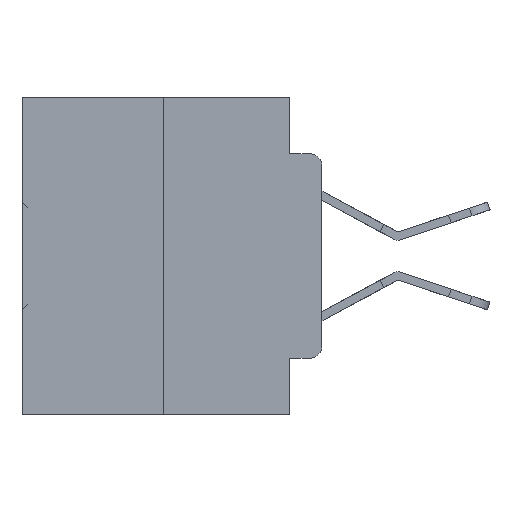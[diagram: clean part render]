
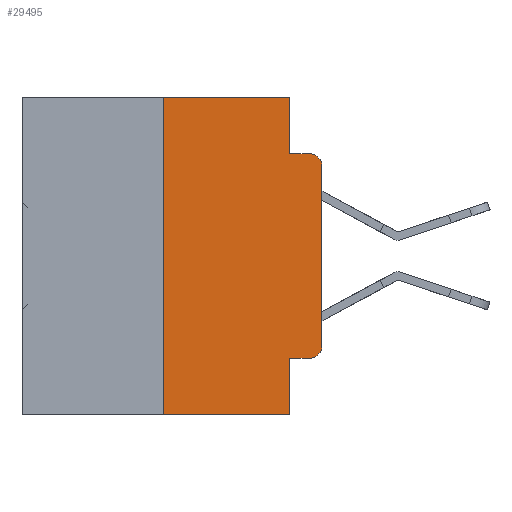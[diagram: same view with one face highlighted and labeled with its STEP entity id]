
A CAD part, left-side view. The second image highlights one B-rep face of the part: STEP entity #29495.
In plain terms, the highlighted planar face has unit normal (-1, 0, 0).
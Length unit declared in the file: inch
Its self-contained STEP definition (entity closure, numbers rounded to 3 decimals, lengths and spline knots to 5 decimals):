
#319 = CARTESIAN_POINT ( 'NONE',  ( 0., 0.051, -0.5 ) ) ;
#462 = VERTEX_POINT ( 'NONE', #13307 ) ;
#950 = VERTEX_POINT ( 'NONE', #319 ) ;
#994 = DIRECTION ( 'NONE',  ( -1., 0., 0. ) ) ;
#1073 = EDGE_CURVE ( 'NONE', #1908, #5815, #4801, .T. ) ;
#1793 = EDGE_CURVE ( 'NONE', #462, #9292, #20117, .T. ) ;
#1815 = LINE ( 'NONE', #3120, #23038 ) ;
#1858 = VERTEX_POINT ( 'NONE', #3463 ) ;
#1908 = VERTEX_POINT ( 'NONE', #36697 ) ;
#2003 = CARTESIAN_POINT ( 'NONE',  ( 0., 0.02, -0.4115 ) ) ;
#2181 = EDGE_CURVE ( 'NONE', #5815, #10513, #35860, .T. ) ;
#3120 = CARTESIAN_POINT ( 'NONE',  ( 0., 0.473, -0.5 ) ) ;
#3243 = CARTESIAN_POINT ( 'NONE',  ( 0., 0.02, -0.3915 ) ) ;
#3463 = CARTESIAN_POINT ( 'NONE',  ( 0., 0., -0.1085 ) ) ;
#3665 = CARTESIAN_POINT ( 'NONE',  ( 0., 0.051, -0.4115 ) ) ;
#3988 = DIRECTION ( 'NONE',  ( 0., 0., 1. ) ) ;
#4154 = LINE ( 'NONE', #35798, #26167 ) ;
#4536 = VECTOR ( 'NONE', #30514, 39.37008 ) ;
#4801 = LINE ( 'NONE', #12631, #35248 ) ;
#5329 = LINE ( 'NONE', #26248, #19744 ) ;
#5815 = VERTEX_POINT ( 'NONE', #7677 ) ;
#6037 = DIRECTION ( 'NONE',  ( 0., -1., 0. ) ) ;
#6159 = DIRECTION ( 'NONE',  ( 0., 0., -1. ) ) ;
#7382 = CARTESIAN_POINT ( 'NONE',  ( 0., 0., -0.3915 ) ) ;
#7677 = CARTESIAN_POINT ( 'NONE',  ( 0., 0.25, 0. ) ) ;
#7715 = CIRCLE ( 'NONE', #22356, 0.02 ) ;
#7912 = EDGE_CURVE ( 'NONE', #10513, #11655, #4154, .T. ) ;
#8356 = CARTESIAN_POINT ( 'NONE',  ( 0., 0.051, 0. ) ) ;
#9292 = VERTEX_POINT ( 'NONE', #2003 ) ;
#10027 = LINE ( 'NONE', #8356, #32860 ) ;
#10513 = VERTEX_POINT ( 'NONE', #33299 ) ;
#10878 = ORIENTED_EDGE ( 'NONE', *, *, #2181, .F. ) ;
#11516 = CARTESIAN_POINT ( 'NONE',  ( 0., 0.051, -0.0885 ) ) ;
#11655 = VERTEX_POINT ( 'NONE', #11516 ) ;
#11855 = ORIENTED_EDGE ( 'NONE', *, *, #34479, .T. ) ;
#11973 = DIRECTION ( 'NONE',  ( 0., 0., 1. ) ) ;
#12333 = ORIENTED_EDGE ( 'NONE', *, *, #1073, .F. ) ;
#12481 = VECTOR ( 'NONE', #24177, 39.37008 ) ;
#12631 = CARTESIAN_POINT ( 'NONE',  ( 0., 0.25, 0. ) ) ;
#13307 = CARTESIAN_POINT ( 'NONE',  ( 0., 0.051, -0.4115 ) ) ;
#13730 = CARTESIAN_POINT ( 'NONE',  ( 0., 0.051, -0.0885 ) ) ;
#14408 = EDGE_LOOP ( 'NONE', ( #31384, #11855, #27970, #23119, #10878, #12333, #22554, #16230, #30542, #15329 ) ) ;
#14472 = FACE_OUTER_BOUND ( 'NONE', #14408, .T. ) ;
#14640 = EDGE_CURVE ( 'NONE', #11655, #15395, #29406, .T. ) ;
#14835 = DIRECTION ( 'NONE',  ( 1., 0., 0. ) ) ;
#15329 = ORIENTED_EDGE ( 'NONE', *, *, #29477, .T. ) ;
#15395 = VERTEX_POINT ( 'NONE', #28304 ) ;
#16230 = ORIENTED_EDGE ( 'NONE', *, *, #28770, .F. ) ;
#16600 = DIRECTION ( 'NONE',  ( 0., -1., 0. ) ) ;
#17180 = AXIS2_PLACEMENT_3D ( 'NONE', #18280, #994, #21189 ) ;
#18153 = VERTEX_POINT ( 'NONE', #7382 ) ;
#18280 = CARTESIAN_POINT ( 'NONE',  ( 0., 0.02, -0.1085 ) ) ;
#18786 = DIRECTION ( 'NONE',  ( 0., 0., -1. ) ) ;
#19744 = VECTOR ( 'NONE', #11973, 39.37008 ) ;
#20117 = LINE ( 'NONE', #3665, #12481 ) ;
#21189 = DIRECTION ( 'NONE',  ( 0., 0., -1. ) ) ;
#22340 = EDGE_CURVE ( 'NONE', #18153, #1858, #5329, .T. ) ;
#22356 = AXIS2_PLACEMENT_3D ( 'NONE', #3243, #23403, #6159 ) ;
#22554 = ORIENTED_EDGE ( 'NONE', *, *, #29467, .T. ) ;
#22942 = CIRCLE ( 'NONE', #17180, 0.02 ) ;
#23038 = VECTOR ( 'NONE', #6037, 39.37008 ) ;
#23119 = ORIENTED_EDGE ( 'NONE', *, *, #7912, .F. ) ;
#23403 = DIRECTION ( 'NONE',  ( -1., 0., 0. ) ) ;
#24177 = DIRECTION ( 'NONE',  ( 0., -1., 0. ) ) ;
#25536 = DIRECTION ( 'NONE',  ( 0., 0., -1. ) ) ;
#26167 = VECTOR ( 'NONE', #18786, 39.37008 ) ;
#26241 = CARTESIAN_POINT ( 'NONE',  ( 0., 0.473, 0. ) ) ;
#26248 = CARTESIAN_POINT ( 'NONE',  ( 0., 0., 0. ) ) ;
#27970 = ORIENTED_EDGE ( 'NONE', *, *, #14640, .F. ) ;
#28304 = CARTESIAN_POINT ( 'NONE',  ( 0., 0.02, -0.0885 ) ) ;
#28770 = EDGE_CURVE ( 'NONE', #462, #950, #10027, .T. ) ;
#29406 = LINE ( 'NONE', #13730, #36908 ) ;
#29467 = EDGE_CURVE ( 'NONE', #1908, #950, #1815, .T. ) ;
#29477 = EDGE_CURVE ( 'NONE', #9292, #18153, #7715, .T. ) ;
#29495 = ADVANCED_FACE ( 'NONE', ( #14472 ), #31972, .F. ) ;
#30514 = DIRECTION ( 'NONE',  ( 0., -1., 0. ) ) ;
#30542 = ORIENTED_EDGE ( 'NONE', *, *, #1793, .T. ) ;
#31384 = ORIENTED_EDGE ( 'NONE', *, *, #22340, .T. ) ;
#31972 = PLANE ( 'NONE',  #33787 ) ;
#32860 = VECTOR ( 'NONE', #25536, 39.37008 ) ;
#33299 = CARTESIAN_POINT ( 'NONE',  ( 0., 0.051, 0. ) ) ;
#33787 = AXIS2_PLACEMENT_3D ( 'NONE', #26241, #14835, #34806 ) ;
#34479 = EDGE_CURVE ( 'NONE', #1858, #15395, #22942, .T. ) ;
#34806 = DIRECTION ( 'NONE',  ( 0., 0., -1. ) ) ;
#35248 = VECTOR ( 'NONE', #3988, 39.37008 ) ;
#35725 = CARTESIAN_POINT ( 'NONE',  ( 0., 0.473, 0. ) ) ;
#35798 = CARTESIAN_POINT ( 'NONE',  ( 0., 0.051, 0. ) ) ;
#35860 = LINE ( 'NONE', #35725, #4536 ) ;
#36697 = CARTESIAN_POINT ( 'NONE',  ( 0., 0.25, -0.5 ) ) ;
#36908 = VECTOR ( 'NONE', #16600, 39.37008 ) ;
